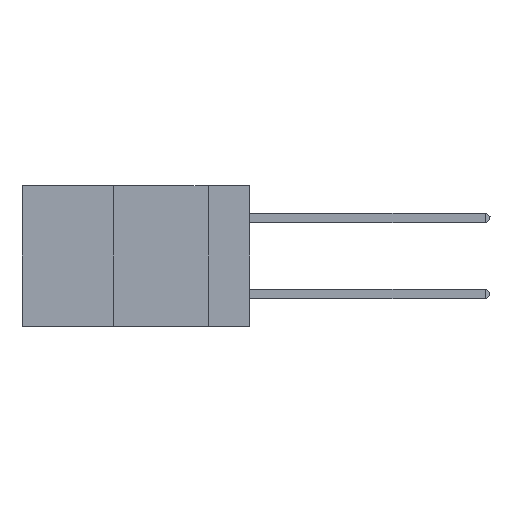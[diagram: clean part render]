
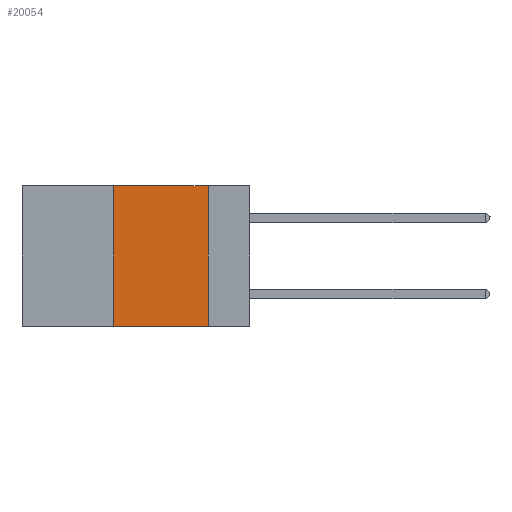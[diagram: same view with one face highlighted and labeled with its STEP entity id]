
A CAD part, left-side view. The second image highlights one B-rep face of the part: STEP entity #20054.
In plain terms, the highlighted planar face has unit normal (-1, 0, 0).
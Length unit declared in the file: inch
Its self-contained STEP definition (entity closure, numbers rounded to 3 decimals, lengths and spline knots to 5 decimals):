
#571 = CARTESIAN_POINT ( 'NONE',  ( 0., 0.36, -0.37 ) ) ;
#1082 = VERTEX_POINT ( 'NONE', #20131 ) ;
#1583 = EDGE_LOOP ( 'NONE', ( #6349, #18223, #23970, #13960 ) ) ;
#4203 = LINE ( 'NONE', #6481, #21639 ) ;
#4214 = LINE ( 'NONE', #14641, #8437 ) ;
#4248 = AXIS2_PLACEMENT_3D ( 'NONE', #6890, #21301, #21576 ) ;
#6349 = ORIENTED_EDGE ( 'NONE', *, *, #18452, .F. ) ;
#6481 = CARTESIAN_POINT ( 'NONE',  ( 0., 0.6, -0.37 ) ) ;
#6750 = PLANE ( 'NONE',  #4248 ) ;
#6890 = CARTESIAN_POINT ( 'NONE',  ( 0., 0.6, 0. ) ) ;
#8276 = DIRECTION ( 'NONE',  ( 0., 0., 1. ) ) ;
#8351 = DIRECTION ( 'NONE',  ( 0., -1., 0. ) ) ;
#8437 = VECTOR ( 'NONE', #20376, 39.37008 ) ;
#10468 = DIRECTION ( 'NONE',  ( 0., -1., 0. ) ) ;
#11557 = EDGE_CURVE ( 'NONE', #12084, #19890, #4203, .T. ) ;
#12084 = VERTEX_POINT ( 'NONE', #571 ) ;
#13149 = FACE_OUTER_BOUND ( 'NONE', #1583, .T. ) ;
#13892 = LINE ( 'NONE', #22302, #19855 ) ;
#13960 = ORIENTED_EDGE ( 'NONE', *, *, #11557, .T. ) ;
#14126 = EDGE_CURVE ( 'NONE', #12084, #21175, #13892, .T. ) ;
#14466 = CARTESIAN_POINT ( 'NONE',  ( 0., 0.6, 0. ) ) ;
#14476 = VECTOR ( 'NONE', #10468, 39.37008 ) ;
#14641 = CARTESIAN_POINT ( 'NONE',  ( 0., 0.11, 0. ) ) ;
#18223 = ORIENTED_EDGE ( 'NONE', *, *, #20317, .F. ) ;
#18452 = EDGE_CURVE ( 'NONE', #1082, #19890, #4214, .T. ) ;
#19855 = VECTOR ( 'NONE', #8276, 39.37008 ) ;
#19890 = VERTEX_POINT ( 'NONE', #25065 ) ;
#20054 = ADVANCED_FACE ( 'NONE', ( #13149 ), #6750, .F. ) ;
#20131 = CARTESIAN_POINT ( 'NONE',  ( 0., 0.11, 0. ) ) ;
#20317 = EDGE_CURVE ( 'NONE', #21175, #1082, #20345, .T. ) ;
#20345 = LINE ( 'NONE', #14466, #14476 ) ;
#20376 = DIRECTION ( 'NONE',  ( 0., 0., -1. ) ) ;
#21175 = VERTEX_POINT ( 'NONE', #22696 ) ;
#21301 = DIRECTION ( 'NONE',  ( 1., 0., 0. ) ) ;
#21576 = DIRECTION ( 'NONE',  ( 0., 0., -1. ) ) ;
#21639 = VECTOR ( 'NONE', #8351, 39.37008 ) ;
#22302 = CARTESIAN_POINT ( 'NONE',  ( 0., 0.36, 0. ) ) ;
#22696 = CARTESIAN_POINT ( 'NONE',  ( 0., 0.36, 0. ) ) ;
#23970 = ORIENTED_EDGE ( 'NONE', *, *, #14126, .F. ) ;
#25065 = CARTESIAN_POINT ( 'NONE',  ( 0., 0.11, -0.37 ) ) ;
